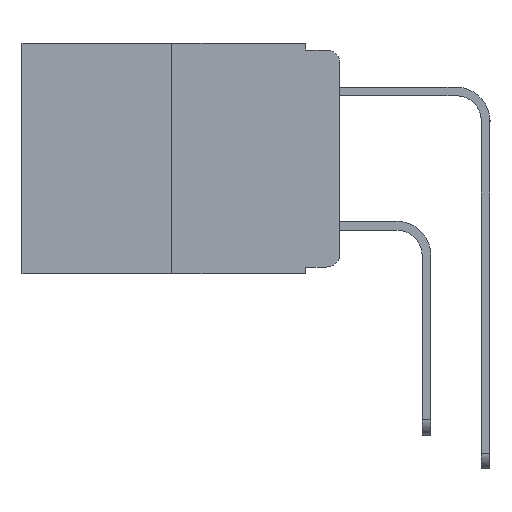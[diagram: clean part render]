
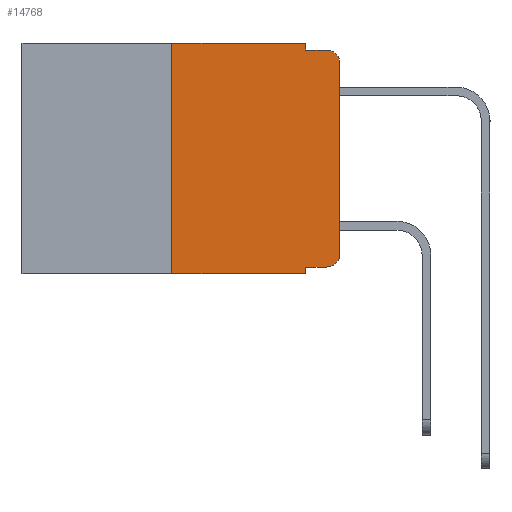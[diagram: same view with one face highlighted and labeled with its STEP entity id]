
A CAD part, left-side view. The second image highlights one B-rep face of the part: STEP entity #14768.
In plain terms, the highlighted planar face has unit normal (-1, 0, 0).
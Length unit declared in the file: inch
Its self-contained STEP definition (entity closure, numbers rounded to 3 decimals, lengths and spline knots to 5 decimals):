
#142 = DIRECTION ( 'NONE',  ( -1., 0., 0. ) ) ;
#180 = ORIENTED_EDGE ( 'NONE', *, *, #13351, .T. ) ;
#460 = EDGE_CURVE ( 'NONE', #8754, #17712, #15657, .T. ) ;
#641 = AXIS2_PLACEMENT_3D ( 'NONE', #7465, #18965, #9159 ) ;
#906 = CARTESIAN_POINT ( 'NONE',  ( 0., 0.051, 0. ) ) ;
#1386 = VERTEX_POINT ( 'NONE', #21393 ) ;
#1444 = LINE ( 'NONE', #8954, #19188 ) ;
#1506 = DIRECTION ( 'NONE',  ( 0., 0., -1. ) ) ;
#1527 = ORIENTED_EDGE ( 'NONE', *, *, #8271, .F. ) ;
#1640 = LINE ( 'NONE', #2592, #19373 ) ;
#1646 = EDGE_CURVE ( 'NONE', #17712, #5615, #3932, .T. ) ;
#1962 = FACE_OUTER_BOUND ( 'NONE', #2593, .T. ) ;
#2010 = AXIS2_PLACEMENT_3D ( 'NONE', #14266, #4295, #15920 ) ;
#2122 = ORIENTED_EDGE ( 'NONE', *, *, #15585, .T. ) ;
#2193 = VERTEX_POINT ( 'NONE', #12013 ) ;
#2546 = PLANE ( 'NONE',  #2010 ) ;
#2592 = CARTESIAN_POINT ( 'NONE',  ( 0., 0.473, -0.343 ) ) ;
#2593 = EDGE_LOOP ( 'NONE', ( #9148, #18843, #8827, #8992, #1527, #7701, #18021, #2948, #2122, #180 ) ) ;
#2948 = ORIENTED_EDGE ( 'NONE', *, *, #16665, .F. ) ;
#3932 = LINE ( 'NONE', #20479, #20947 ) ;
#4295 = DIRECTION ( 'NONE',  ( 1., 0., 0. ) ) ;
#4468 = VERTEX_POINT ( 'NONE', #19759 ) ;
#4487 = CARTESIAN_POINT ( 'NONE',  ( 0., 0.02, -0.01 ) ) ;
#5615 = VERTEX_POINT ( 'NONE', #4487 ) ;
#6289 = EDGE_CURVE ( 'NONE', #12586, #5615, #8354, .T. ) ;
#7412 = EDGE_CURVE ( 'NONE', #16648, #12586, #16793, .T. ) ;
#7465 = CARTESIAN_POINT ( 'NONE',  ( 0., 0.02, -0.313 ) ) ;
#7701 = ORIENTED_EDGE ( 'NONE', *, *, #19921, .F. ) ;
#8271 = EDGE_CURVE ( 'NONE', #19351, #8754, #1444, .T. ) ;
#8354 = CIRCLE ( 'NONE', #16456, 0.02 ) ;
#8754 = VERTEX_POINT ( 'NONE', #20098 ) ;
#8827 = ORIENTED_EDGE ( 'NONE', *, *, #1646, .F. ) ;
#8954 = CARTESIAN_POINT ( 'NONE',  ( 0., 0.473, 0. ) ) ;
#8992 = ORIENTED_EDGE ( 'NONE', *, *, #460, .F. ) ;
#9021 = DIRECTION ( 'NONE',  ( 0., -1., 0. ) ) ;
#9148 = ORIENTED_EDGE ( 'NONE', *, *, #7412, .T. ) ;
#9159 = DIRECTION ( 'NONE',  ( 0., 0., -1. ) ) ;
#9334 = LINE ( 'NONE', #11621, #18056 ) ;
#9842 = DIRECTION ( 'NONE',  ( 0., 0., 1. ) ) ;
#10388 = CARTESIAN_POINT ( 'NONE',  ( 0., 0.02, -0.03 ) ) ;
#10613 = DIRECTION ( 'NONE',  ( 0., -1., 0. ) ) ;
#11059 = CARTESIAN_POINT ( 'NONE',  ( 0., 0.051, -0.01 ) ) ;
#11226 = CARTESIAN_POINT ( 'NONE',  ( 0., 0.25, 0. ) ) ;
#11336 = CARTESIAN_POINT ( 'NONE',  ( 0., 0.051, -0.333 ) ) ;
#11481 = CARTESIAN_POINT ( 'NONE',  ( 0., 0., 0. ) ) ;
#11533 = CARTESIAN_POINT ( 'NONE',  ( 0., 0.25, 0. ) ) ;
#11621 = CARTESIAN_POINT ( 'NONE',  ( 0., 0.051, 0. ) ) ;
#11935 = VECTOR ( 'NONE', #12989, 39.37008 ) ;
#12013 = CARTESIAN_POINT ( 'NONE',  ( 0., 0.25, -0.343 ) ) ;
#12022 = DIRECTION ( 'NONE',  ( 0., 0., -1. ) ) ;
#12310 = CIRCLE ( 'NONE', #641, 0.02 ) ;
#12440 = LINE ( 'NONE', #11336, #11935 ) ;
#12586 = VERTEX_POINT ( 'NONE', #17077 ) ;
#12989 = DIRECTION ( 'NONE',  ( 0., -1., 0. ) ) ;
#13351 = EDGE_CURVE ( 'NONE', #1386, #16648, #12310, .T. ) ;
#14266 = CARTESIAN_POINT ( 'NONE',  ( 0., 0.473, 0. ) ) ;
#14411 = DIRECTION ( 'NONE',  ( 0., 0., -1. ) ) ;
#14637 = VECTOR ( 'NONE', #17763, 39.37008 ) ;
#14768 = ADVANCED_FACE ( 'NONE', ( #1962 ), #2546, .F. ) ;
#14824 = CARTESIAN_POINT ( 'NONE',  ( 0., 0., -0.313 ) ) ;
#15447 = EDGE_CURVE ( 'NONE', #2193, #4468, #1640, .T. ) ;
#15585 = EDGE_CURVE ( 'NONE', #15768, #1386, #12440, .T. ) ;
#15657 = LINE ( 'NONE', #906, #19452 ) ;
#15768 = VERTEX_POINT ( 'NONE', #18289 ) ;
#15920 = DIRECTION ( 'NONE',  ( 0., 0., -1. ) ) ;
#16303 = VECTOR ( 'NONE', #9842, 39.37008 ) ;
#16456 = AXIS2_PLACEMENT_3D ( 'NONE', #10388, #142, #12022 ) ;
#16648 = VERTEX_POINT ( 'NONE', #14824 ) ;
#16665 = EDGE_CURVE ( 'NONE', #15768, #4468, #9334, .T. ) ;
#16793 = LINE ( 'NONE', #11481, #16303 ) ;
#17077 = CARTESIAN_POINT ( 'NONE',  ( 0., 0., -0.03 ) ) ;
#17507 = DIRECTION ( 'NONE',  ( 0., -1., 0. ) ) ;
#17712 = VERTEX_POINT ( 'NONE', #11059 ) ;
#17763 = DIRECTION ( 'NONE',  ( 0., 0., 1. ) ) ;
#18021 = ORIENTED_EDGE ( 'NONE', *, *, #15447, .T. ) ;
#18056 = VECTOR ( 'NONE', #1506, 39.37008 ) ;
#18289 = CARTESIAN_POINT ( 'NONE',  ( 0., 0.051, -0.333 ) ) ;
#18843 = ORIENTED_EDGE ( 'NONE', *, *, #6289, .T. ) ;
#18958 = LINE ( 'NONE', #11226, #14637 ) ;
#18965 = DIRECTION ( 'NONE',  ( -1., 0., 0. ) ) ;
#19188 = VECTOR ( 'NONE', #9021, 39.37008 ) ;
#19351 = VERTEX_POINT ( 'NONE', #11533 ) ;
#19373 = VECTOR ( 'NONE', #17507, 39.37008 ) ;
#19452 = VECTOR ( 'NONE', #14411, 39.37008 ) ;
#19759 = CARTESIAN_POINT ( 'NONE',  ( 0., 0.051, -0.343 ) ) ;
#19921 = EDGE_CURVE ( 'NONE', #2193, #19351, #18958, .T. ) ;
#20098 = CARTESIAN_POINT ( 'NONE',  ( 0., 0.051, 0. ) ) ;
#20479 = CARTESIAN_POINT ( 'NONE',  ( 0., 0.051, -0.01 ) ) ;
#20947 = VECTOR ( 'NONE', #10613, 39.37008 ) ;
#21393 = CARTESIAN_POINT ( 'NONE',  ( 0., 0.02, -0.333 ) ) ;
